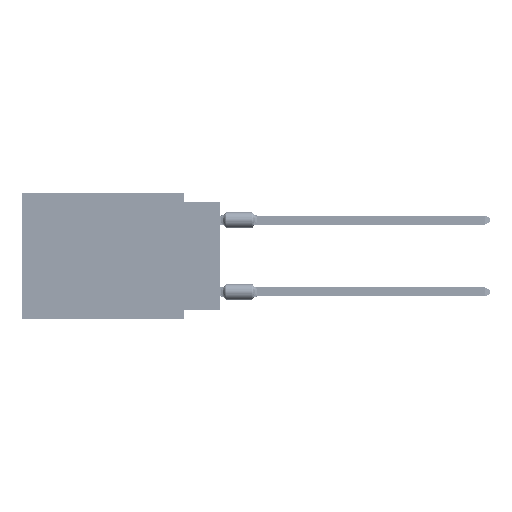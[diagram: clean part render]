
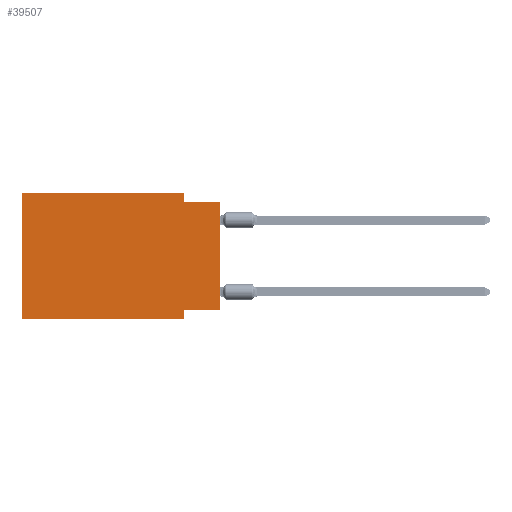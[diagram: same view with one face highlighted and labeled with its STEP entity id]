
A CAD part, left-side view. The second image highlights one B-rep face of the part: STEP entity #39507.
In plain terms, the highlighted planar face has unit normal (-1, 0, 0).
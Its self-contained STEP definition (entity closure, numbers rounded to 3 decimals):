
#450 = ORIENTED_EDGE ( 'NONE', *, *, #39054, .F. ) ;
#1007 = CARTESIAN_POINT ( 'NONE',  ( 0., 0., -0.635 ) ) ;
#1681 = DIRECTION ( 'NONE',  ( 0., 0., -1. ) ) ;
#2924 = DIRECTION ( 'NONE',  ( 0., 0., -1. ) ) ;
#3877 = CARTESIAN_POINT ( 'NONE',  ( 0., 13.97, -8.89 ) ) ;
#4504 = EDGE_CURVE ( 'NONE', #18832, #15600, #69947, .T. ) ;
#5670 = LINE ( 'NONE', #54631, #31462 ) ;
#8592 = ORIENTED_EDGE ( 'NONE', *, *, #37328, .F. ) ;
#8777 = LINE ( 'NONE', #24881, #9201 ) ;
#9201 = VECTOR ( 'NONE', #29570, 1000. ) ;
#9415 = CARTESIAN_POINT ( 'NONE',  ( 0., 2.54, -8.89 ) ) ;
#10457 = VECTOR ( 'NONE', #53194, 1000. ) ;
#12304 = CARTESIAN_POINT ( 'NONE',  ( 0., 2.54, -8.255 ) ) ;
#14599 = CARTESIAN_POINT ( 'NONE',  ( 0., 2.54, -8.89 ) ) ;
#15600 = VERTEX_POINT ( 'NONE', #33869 ) ;
#15692 = EDGE_LOOP ( 'NONE', ( #32584, #22279, #59030, #450, #34426, #45486, #57062, #8592 ) ) ;
#17027 = DIRECTION ( 'NONE',  ( 0., 0., 1. ) ) ;
#18025 = CARTESIAN_POINT ( 'NONE',  ( 0., 13.97, 0. ) ) ;
#18832 = VERTEX_POINT ( 'NONE', #21116 ) ;
#20411 = VECTOR ( 'NONE', #25667, 1000. ) ;
#21116 = CARTESIAN_POINT ( 'NONE',  ( 0., 0., -8.255 ) ) ;
#22279 = ORIENTED_EDGE ( 'NONE', *, *, #52579, .F. ) ;
#23969 = VECTOR ( 'NONE', #17027, 1000. ) ;
#24881 = CARTESIAN_POINT ( 'NONE',  ( 0., 0., -8.255 ) ) ;
#25667 = DIRECTION ( 'NONE',  ( 0., -1., 0. ) ) ;
#27399 = DIRECTION ( 'NONE',  ( 0., -1., 0. ) ) ;
#29570 = DIRECTION ( 'NONE',  ( 0., 1., 0. ) ) ;
#29744 = EDGE_CURVE ( 'NONE', #51582, #36808, #37812, .T. ) ;
#31024 = EDGE_CURVE ( 'NONE', #68753, #53539, #5670, .T. ) ;
#31462 = VECTOR ( 'NONE', #1681, 1000. ) ;
#32584 = ORIENTED_EDGE ( 'NONE', *, *, #4504, .T. ) ;
#32709 = DIRECTION ( 'NONE',  ( 0., 0., 1. ) ) ;
#32743 = CARTESIAN_POINT ( 'NONE',  ( 0., 13.97, 0. ) ) ;
#33766 = LINE ( 'NONE', #18025, #36386 ) ;
#33869 = CARTESIAN_POINT ( 'NONE',  ( 0., 0., -0.635 ) ) ;
#34426 = ORIENTED_EDGE ( 'NONE', *, *, #49599, .F. ) ;
#35468 = FACE_OUTER_BOUND ( 'NONE', #15692, .T. ) ;
#36386 = VECTOR ( 'NONE', #27399, 1000. ) ;
#36808 = VERTEX_POINT ( 'NONE', #9415 ) ;
#37328 = EDGE_CURVE ( 'NONE', #18832, #37757, #8777, .T. ) ;
#37757 = VERTEX_POINT ( 'NONE', #12304 ) ;
#37812 = LINE ( 'NONE', #3877, #20411 ) ;
#39054 = EDGE_CURVE ( 'NONE', #70158, #68753, #33766, .T. ) ;
#39507 = ADVANCED_FACE ( 'NONE', ( #35468 ), #39758, .F. ) ;
#39758 = PLANE ( 'NONE',  #40918 ) ;
#39951 = LINE ( 'NONE', #1007, #58983 ) ;
#40293 = CARTESIAN_POINT ( 'NONE',  ( 0., 2.54, 0. ) ) ;
#40297 = DIRECTION ( 'NONE',  ( 0., -1., 0. ) ) ;
#40918 = AXIS2_PLACEMENT_3D ( 'NONE', #45840, #46183, #2924 ) ;
#45486 = ORIENTED_EDGE ( 'NONE', *, *, #29744, .T. ) ;
#45840 = CARTESIAN_POINT ( 'NONE',  ( 0., 13.97, 0. ) ) ;
#46183 = DIRECTION ( 'NONE',  ( 1., 0., 0. ) ) ;
#47610 = CARTESIAN_POINT ( 'NONE',  ( 0., 13.97, -8.89 ) ) ;
#49599 = EDGE_CURVE ( 'NONE', #51582, #70158, #54217, .T. ) ;
#51582 = VERTEX_POINT ( 'NONE', #47610 ) ;
#52579 = EDGE_CURVE ( 'NONE', #53539, #15600, #39951, .T. ) ;
#53194 = DIRECTION ( 'NONE',  ( 0., 0., -1. ) ) ;
#53539 = VERTEX_POINT ( 'NONE', #68983 ) ;
#54187 = CARTESIAN_POINT ( 'NONE',  ( 0., 0., 0. ) ) ;
#54217 = LINE ( 'NONE', #32743, #23969 ) ;
#54631 = CARTESIAN_POINT ( 'NONE',  ( 0., 2.54, 0. ) ) ;
#57062 = ORIENTED_EDGE ( 'NONE', *, *, #61798, .F. ) ;
#58584 = LINE ( 'NONE', #14599, #10457 ) ;
#58983 = VECTOR ( 'NONE', #40297, 1000. ) ;
#59030 = ORIENTED_EDGE ( 'NONE', *, *, #31024, .F. ) ;
#61798 = EDGE_CURVE ( 'NONE', #37757, #36808, #58584, .T. ) ;
#63990 = CARTESIAN_POINT ( 'NONE',  ( 0., 13.97, 0. ) ) ;
#68753 = VERTEX_POINT ( 'NONE', #40293 ) ;
#68983 = CARTESIAN_POINT ( 'NONE',  ( 0., 2.54, -0.635 ) ) ;
#69947 = LINE ( 'NONE', #54187, #70457 ) ;
#70158 = VERTEX_POINT ( 'NONE', #63990 ) ;
#70457 = VECTOR ( 'NONE', #32709, 1000. ) ;
